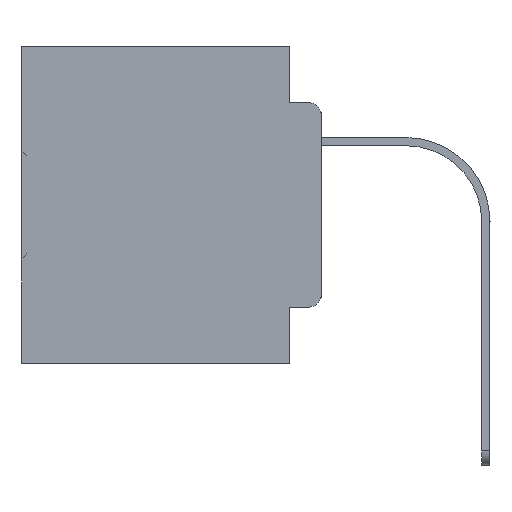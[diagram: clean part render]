
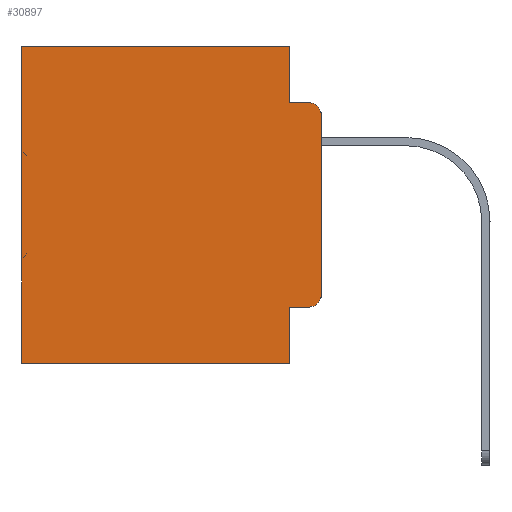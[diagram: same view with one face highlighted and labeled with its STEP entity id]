
A CAD part, left-side view. The second image highlights one B-rep face of the part: STEP entity #30897.
In plain terms, the highlighted planar face has unit normal (-1, 0, 0).
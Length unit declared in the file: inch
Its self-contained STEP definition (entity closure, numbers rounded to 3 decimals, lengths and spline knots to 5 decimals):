
#501 = ORIENTED_EDGE ( 'NONE', *, *, #4941, .T. ) ;
#1028 = LINE ( 'NONE', #4446, #35830 ) ;
#1172 = CARTESIAN_POINT ( 'NONE',  ( 0.298, 0.051, 0. ) ) ;
#2719 = ORIENTED_EDGE ( 'NONE', *, *, #14429, .F. ) ;
#2745 = EDGE_CURVE ( 'NONE', #16260, #30933, #4867, .T. ) ;
#3295 = CARTESIAN_POINT ( 'NONE',  ( 0.298, 0.051, -0.0885 ) ) ;
#3756 = DIRECTION ( 'NONE',  ( 0., 0., -1. ) ) ;
#3911 = CARTESIAN_POINT ( 'NONE',  ( 0.298, 0.473, -0.5 ) ) ;
#4301 = CARTESIAN_POINT ( 'NONE',  ( 0.298, 0.051, 0. ) ) ;
#4446 = CARTESIAN_POINT ( 'NONE',  ( 0.298, 0., 0. ) ) ;
#4502 = EDGE_CURVE ( 'NONE', #14369, #27801, #23810, .T. ) ;
#4776 = DIRECTION ( 'NONE',  ( -1., 0., 0. ) ) ;
#4867 = CIRCLE ( 'NONE', #16411, 0.02 ) ;
#4892 = DIRECTION ( 'NONE',  ( 0., -1., 0. ) ) ;
#4941 = EDGE_CURVE ( 'NONE', #19078, #27801, #31024, .T. ) ;
#4972 = ORIENTED_EDGE ( 'NONE', *, *, #22746, .T. ) ;
#5127 = DIRECTION ( 'NONE',  ( 0., 0., -1. ) ) ;
#5591 = DIRECTION ( 'NONE',  ( 0., -1., 0. ) ) ;
#5617 = CARTESIAN_POINT ( 'NONE',  ( 0.298, 0.02, -0.0885 ) ) ;
#5901 = CARTESIAN_POINT ( 'NONE',  ( 0.298, 0., -0.1085 ) ) ;
#6145 = VERTEX_POINT ( 'NONE', #5901 ) ;
#6191 = VECTOR ( 'NONE', #7479, 39.37008 ) ;
#6605 = LINE ( 'NONE', #1172, #17509 ) ;
#6608 = CARTESIAN_POINT ( 'NONE',  ( 0.298, 0.051, 0. ) ) ;
#6643 = DIRECTION ( 'NONE',  ( 0., 1., 0. ) ) ;
#6776 = DIRECTION ( 'NONE',  ( 0., 0., -1. ) ) ;
#6902 = ORIENTED_EDGE ( 'NONE', *, *, #10428, .F. ) ;
#7479 = DIRECTION ( 'NONE',  ( 0., 0., -1. ) ) ;
#8266 = ORIENTED_EDGE ( 'NONE', *, *, #30182, .T. ) ;
#8983 = ORIENTED_EDGE ( 'NONE', *, *, #30773, .T. ) ;
#10428 = EDGE_CURVE ( 'NONE', #19142, #29800, #17867, .T. ) ;
#10838 = LINE ( 'NONE', #24610, #10936 ) ;
#10936 = VECTOR ( 'NONE', #4892, 39.37008 ) ;
#12256 = AXIS2_PLACEMENT_3D ( 'NONE', #18341, #4776, #31767 ) ;
#12668 = EDGE_CURVE ( 'NONE', #6145, #30933, #1028, .T. ) ;
#12723 = ORIENTED_EDGE ( 'NONE', *, *, #4502, .F. ) ;
#13641 = DIRECTION ( 'NONE',  ( 0., 0., -1. ) ) ;
#14304 = ORIENTED_EDGE ( 'NONE', *, *, #12668, .F. ) ;
#14369 = VERTEX_POINT ( 'NONE', #16921 ) ;
#14429 = EDGE_CURVE ( 'NONE', #29762, #14369, #6605, .T. ) ;
#15620 = CARTESIAN_POINT ( 'NONE',  ( 0.298, 0.02, -0.4115 ) ) ;
#15794 = CARTESIAN_POINT ( 'NONE',  ( 0.298, 0.473, 0. ) ) ;
#16260 = VERTEX_POINT ( 'NONE', #15620 ) ;
#16411 = AXIS2_PLACEMENT_3D ( 'NONE', #21606, #26699, #5127 ) ;
#16467 = LINE ( 'NONE', #33131, #33115 ) ;
#16921 = CARTESIAN_POINT ( 'NONE',  ( 0.298, 0.051, -0.5 ) ) ;
#17509 = VECTOR ( 'NONE', #6776, 39.37008 ) ;
#17573 = VECTOR ( 'NONE', #18229, 39.37008 ) ;
#17867 = LINE ( 'NONE', #4301, #17573 ) ;
#18229 = DIRECTION ( 'NONE',  ( 0., 0., -1. ) ) ;
#18341 = CARTESIAN_POINT ( 'NONE',  ( 0.298, 0.02, -0.1085 ) ) ;
#18364 = CARTESIAN_POINT ( 'NONE',  ( 0.298, 0., -0.5 ) ) ;
#18712 = DIRECTION ( 'NONE',  ( 1., 0., 0. ) ) ;
#18878 = FACE_OUTER_BOUND ( 'NONE', #33805, .T. ) ;
#19078 = VERTEX_POINT ( 'NONE', #31420 ) ;
#19142 = VERTEX_POINT ( 'NONE', #6608 ) ;
#20338 = CIRCLE ( 'NONE', #12256, 0.02 ) ;
#20569 = CARTESIAN_POINT ( 'NONE',  ( 0.298, 0., 0. ) ) ;
#20995 = VERTEX_POINT ( 'NONE', #5617 ) ;
#21419 = CARTESIAN_POINT ( 'NONE',  ( 0.298, 0., 0. ) ) ;
#21606 = CARTESIAN_POINT ( 'NONE',  ( 0.298, 0.02, -0.3915 ) ) ;
#21771 = CARTESIAN_POINT ( 'NONE',  ( 0.298, 0., -0.3915 ) ) ;
#22746 = EDGE_CURVE ( 'NONE', #29762, #16260, #10838, .T. ) ;
#23182 = VECTOR ( 'NONE', #6643, 39.37008 ) ;
#23810 = LINE ( 'NONE', #18364, #30521 ) ;
#24164 = DIRECTION ( 'NONE',  ( 0., 1., 0. ) ) ;
#24610 = CARTESIAN_POINT ( 'NONE',  ( 0.298, 0.051, -0.4115 ) ) ;
#25482 = LINE ( 'NONE', #20569, #23182 ) ;
#26699 = DIRECTION ( 'NONE',  ( -1., 0., 0. ) ) ;
#27801 = VERTEX_POINT ( 'NONE', #3911 ) ;
#28107 = CARTESIAN_POINT ( 'NONE',  ( 0.298, 0.051, -0.4115 ) ) ;
#29640 = ORIENTED_EDGE ( 'NONE', *, *, #2745, .T. ) ;
#29762 = VERTEX_POINT ( 'NONE', #28107 ) ;
#29800 = VERTEX_POINT ( 'NONE', #3295 ) ;
#30182 = EDGE_CURVE ( 'NONE', #19142, #19078, #25482, .T. ) ;
#30521 = VECTOR ( 'NONE', #24164, 39.37008 ) ;
#30773 = EDGE_CURVE ( 'NONE', #6145, #20995, #20338, .T. ) ;
#30897 = ADVANCED_FACE ( 'NONE', ( #18878 ), #35739, .F. ) ;
#30933 = VERTEX_POINT ( 'NONE', #21771 ) ;
#31024 = LINE ( 'NONE', #15794, #6191 ) ;
#31339 = AXIS2_PLACEMENT_3D ( 'NONE', #21419, #18712, #13641 ) ;
#31420 = CARTESIAN_POINT ( 'NONE',  ( 0.298, 0.473, 0. ) ) ;
#31767 = DIRECTION ( 'NONE',  ( 0., 0., -1. ) ) ;
#33115 = VECTOR ( 'NONE', #5591, 39.37008 ) ;
#33131 = CARTESIAN_POINT ( 'NONE',  ( 0.298, 0.051, -0.0885 ) ) ;
#33805 = EDGE_LOOP ( 'NONE', ( #14304, #8983, #35688, #6902, #8266, #501, #12723, #2719, #4972, #29640 ) ) ;
#35088 = EDGE_CURVE ( 'NONE', #29800, #20995, #16467, .T. ) ;
#35688 = ORIENTED_EDGE ( 'NONE', *, *, #35088, .F. ) ;
#35739 = PLANE ( 'NONE',  #31339 ) ;
#35830 = VECTOR ( 'NONE', #3756, 39.37008 ) ;
